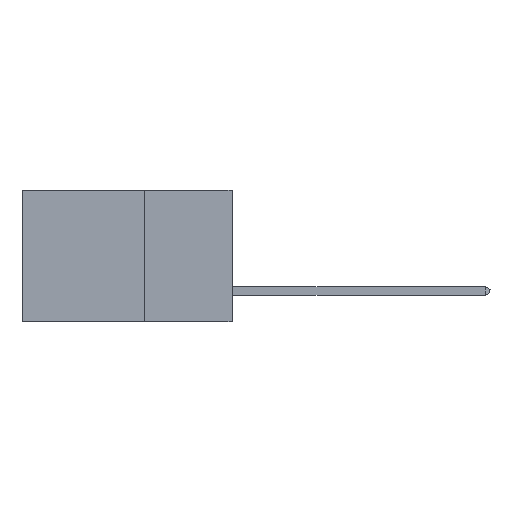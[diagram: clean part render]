
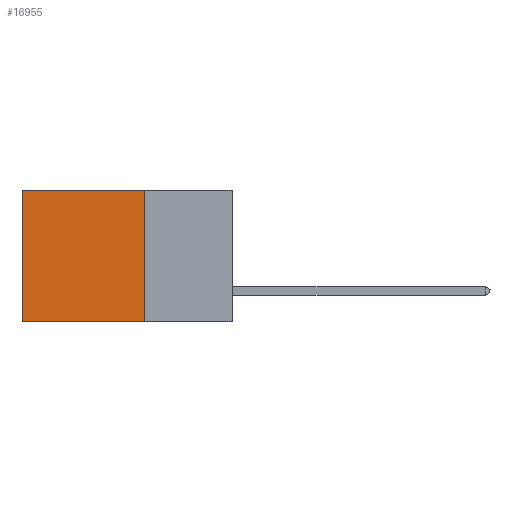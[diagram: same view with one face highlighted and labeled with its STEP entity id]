
A CAD part, left-side view. The second image highlights one B-rep face of the part: STEP entity #16955.
In plain terms, the highlighted planar face has unit normal (-1, 0, 0).
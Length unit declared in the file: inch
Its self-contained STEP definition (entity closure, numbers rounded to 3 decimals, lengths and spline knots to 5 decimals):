
#385 = LINE ( 'NONE', #17133, #5676 ) ;
#495 = VECTOR ( 'NONE', #5053, 39.37008 ) ;
#1203 = VERTEX_POINT ( 'NONE', #7724 ) ;
#3518 = CARTESIAN_POINT ( 'NONE',  ( 0.2875, 0.25, 0. ) ) ;
#3709 = ORIENTED_EDGE ( 'NONE', *, *, #10221, .T. ) ;
#3738 = VECTOR ( 'NONE', #10906, 39.37008 ) ;
#4156 = EDGE_CURVE ( 'NONE', #1203, #6466, #14864, .T. ) ;
#4472 = DIRECTION ( 'NONE',  ( 0., 0., -1. ) ) ;
#5053 = DIRECTION ( 'NONE',  ( 0., 1., 0. ) ) ;
#5676 = VECTOR ( 'NONE', #10873, 39.37008 ) ;
#6107 = CARTESIAN_POINT ( 'NONE',  ( 0.2875, 0.25, -0.375 ) ) ;
#6466 = VERTEX_POINT ( 'NONE', #20694 ) ;
#7724 = CARTESIAN_POINT ( 'NONE',  ( 0.2875, 0.25, 0. ) ) ;
#8314 = ORIENTED_EDGE ( 'NONE', *, *, #17229, .F. ) ;
#8578 = EDGE_CURVE ( 'NONE', #1203, #18344, #11058, .T. ) ;
#8881 = CARTESIAN_POINT ( 'NONE',  ( 0.2875, 0.25, -0.375 ) ) ;
#9548 = CARTESIAN_POINT ( 'NONE',  ( 0.2875, 0.25, -0.375 ) ) ;
#9649 = EDGE_LOOP ( 'NONE', ( #3709, #8314, #11686, #19440 ) ) ;
#10221 = EDGE_CURVE ( 'NONE', #6466, #18374, #385, .T. ) ;
#10294 = AXIS2_PLACEMENT_3D ( 'NONE', #9548, #20824, #4472 ) ;
#10873 = DIRECTION ( 'NONE',  ( 0., 0., -1. ) ) ;
#10906 = DIRECTION ( 'NONE',  ( 0., 0., -1. ) ) ;
#11058 = LINE ( 'NONE', #6107, #3738 ) ;
#11686 = ORIENTED_EDGE ( 'NONE', *, *, #8578, .F. ) ;
#11819 = FACE_OUTER_BOUND ( 'NONE', #9649, .T. ) ;
#12446 = CARTESIAN_POINT ( 'NONE',  ( 0.2875, 0.6, -0.375 ) ) ;
#12788 = VECTOR ( 'NONE', #15902, 39.37008 ) ;
#14126 = PLANE ( 'NONE',  #10294 ) ;
#14864 = LINE ( 'NONE', #3518, #495 ) ;
#15902 = DIRECTION ( 'NONE',  ( 0., 1., 0. ) ) ;
#16039 = CARTESIAN_POINT ( 'NONE',  ( 0.2875, 0.25, -0.375 ) ) ;
#16355 = LINE ( 'NONE', #16039, #12788 ) ;
#16955 = ADVANCED_FACE ( 'NONE', ( #11819 ), #14126, .F. ) ;
#17133 = CARTESIAN_POINT ( 'NONE',  ( 0.2875, 0.6, -0.375 ) ) ;
#17229 = EDGE_CURVE ( 'NONE', #18344, #18374, #16355, .T. ) ;
#18344 = VERTEX_POINT ( 'NONE', #8881 ) ;
#18374 = VERTEX_POINT ( 'NONE', #12446 ) ;
#19440 = ORIENTED_EDGE ( 'NONE', *, *, #4156, .T. ) ;
#20694 = CARTESIAN_POINT ( 'NONE',  ( 0.2875, 0.6, 0. ) ) ;
#20824 = DIRECTION ( 'NONE',  ( 1., 0., 0. ) ) ;
